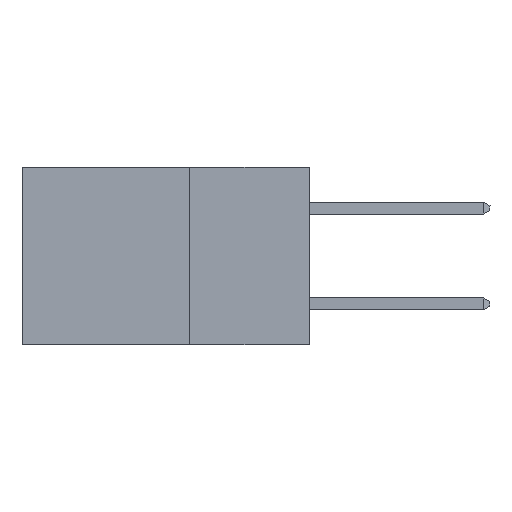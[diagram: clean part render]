
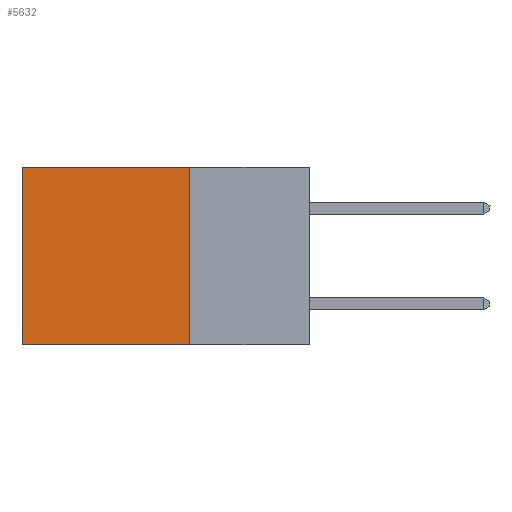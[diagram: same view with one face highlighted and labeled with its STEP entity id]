
A CAD part, left-side view. The second image highlights one B-rep face of the part: STEP entity #5632.
In plain terms, the highlighted planar face has unit normal (-1, 0, 0).
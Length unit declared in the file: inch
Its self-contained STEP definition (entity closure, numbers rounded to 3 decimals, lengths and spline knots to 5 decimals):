
#656 = EDGE_CURVE ( 'NONE', #3845, #3909, #2276, .T. ) ;
#837 = DIRECTION ( 'NONE',  ( 0., 1., 0. ) ) ;
#1488 = CARTESIAN_POINT ( 'NONE',  ( 0.2875, 0.6, -0.37 ) ) ;
#2276 = LINE ( 'NONE', #4119, #8414 ) ;
#2317 = EDGE_CURVE ( 'NONE', #6512, #3845, #9619, .T. ) ;
#3293 = ORIENTED_EDGE ( 'NONE', *, *, #6683, .F. ) ;
#3584 = DIRECTION ( 'NONE',  ( 1., 0., 0. ) ) ;
#3845 = VERTEX_POINT ( 'NONE', #9298 ) ;
#3852 = CARTESIAN_POINT ( 'NONE',  ( 0.2875, 0.25, 0. ) ) ;
#3909 = VERTEX_POINT ( 'NONE', #1488 ) ;
#4053 = ORIENTED_EDGE ( 'NONE', *, *, #656, .T. ) ;
#4119 = CARTESIAN_POINT ( 'NONE',  ( 0.2875, 0.6, 0. ) ) ;
#4184 = AXIS2_PLACEMENT_3D ( 'NONE', #6575, #3584, #6467 ) ;
#4569 = VECTOR ( 'NONE', #4635, 39.37008 ) ;
#4635 = DIRECTION ( 'NONE',  ( 0., 1., 0. ) ) ;
#4660 = FACE_OUTER_BOUND ( 'NONE', #8314, .T. ) ;
#4686 = LINE ( 'NONE', #9739, #6949 ) ;
#5292 = ORIENTED_EDGE ( 'NONE', *, *, #12342, .F. ) ;
#5355 = PLANE ( 'NONE',  #4184 ) ;
#5632 = ADVANCED_FACE ( 'NONE', ( #4660 ), #5355, .F. ) ;
#5896 = VECTOR ( 'NONE', #837, 39.37008 ) ;
#6467 = DIRECTION ( 'NONE',  ( 0., 0., -1. ) ) ;
#6512 = VERTEX_POINT ( 'NONE', #10959 ) ;
#6575 = CARTESIAN_POINT ( 'NONE',  ( 0.2875, 0.25, 0. ) ) ;
#6683 = EDGE_CURVE ( 'NONE', #6512, #8937, #4686, .T. ) ;
#6949 = VECTOR ( 'NONE', #11461, 39.37008 ) ;
#8314 = EDGE_LOOP ( 'NONE', ( #4053, #5292, #3293, #12494 ) ) ;
#8414 = VECTOR ( 'NONE', #11972, 39.37008 ) ;
#8514 = CARTESIAN_POINT ( 'NONE',  ( 0.2875, 0.25, -0.37 ) ) ;
#8937 = VERTEX_POINT ( 'NONE', #9337 ) ;
#9298 = CARTESIAN_POINT ( 'NONE',  ( 0.2875, 0.6, 0. ) ) ;
#9337 = CARTESIAN_POINT ( 'NONE',  ( 0.2875, 0.25, -0.37 ) ) ;
#9619 = LINE ( 'NONE', #3852, #4569 ) ;
#9739 = CARTESIAN_POINT ( 'NONE',  ( 0.2875, 0.25, 0. ) ) ;
#10121 = LINE ( 'NONE', #8514, #5896 ) ;
#10959 = CARTESIAN_POINT ( 'NONE',  ( 0.2875, 0.25, 0. ) ) ;
#11461 = DIRECTION ( 'NONE',  ( 0., 0., -1. ) ) ;
#11972 = DIRECTION ( 'NONE',  ( 0., 0., -1. ) ) ;
#12342 = EDGE_CURVE ( 'NONE', #8937, #3909, #10121, .T. ) ;
#12494 = ORIENTED_EDGE ( 'NONE', *, *, #2317, .T. ) ;
